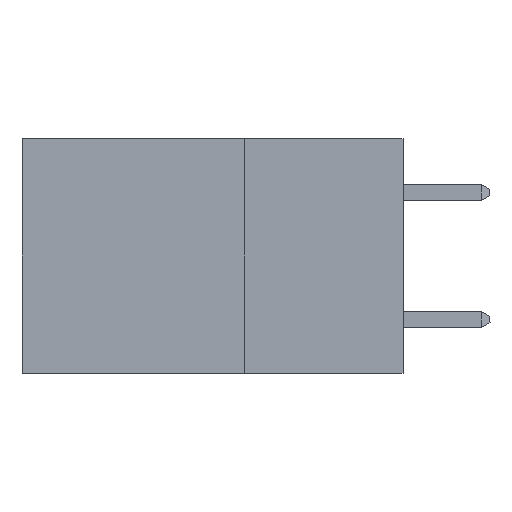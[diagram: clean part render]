
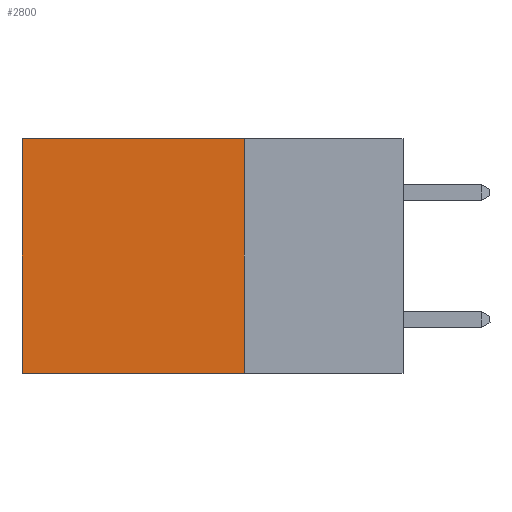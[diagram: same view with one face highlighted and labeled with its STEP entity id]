
A CAD part, left-side view. The second image highlights one B-rep face of the part: STEP entity #2800.
In plain terms, the highlighted planar face has unit normal (-1, 0, 0).
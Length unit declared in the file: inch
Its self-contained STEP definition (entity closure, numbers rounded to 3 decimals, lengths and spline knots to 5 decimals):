
#167 = AXIS2_PLACEMENT_3D ( 'NONE', #10324, #6565, #6544 ) ;
#244 = EDGE_CURVE ( 'NONE', #8905, #12550, #1825, .T. ) ;
#961 = LINE ( 'NONE', #6795, #11125 ) ;
#1372 = DIRECTION ( 'NONE',  ( 0., 1., 0. ) ) ;
#1406 = CARTESIAN_POINT ( 'NONE',  ( 0.2875, 0.25, -0.37 ) ) ;
#1825 = LINE ( 'NONE', #7615, #15183 ) ;
#2068 = ORIENTED_EDGE ( 'NONE', *, *, #244, .F. ) ;
#2527 = EDGE_CURVE ( 'NONE', #4469, #8905, #10467, .T. ) ;
#2800 = ADVANCED_FACE ( 'NONE', ( #6689 ), #5011, .F. ) ;
#3368 = VECTOR ( 'NONE', #6262, 39.37008 ) ;
#3665 = EDGE_LOOP ( 'NONE', ( #4724, #2068, #9142, #15760 ) ) ;
#4469 = VERTEX_POINT ( 'NONE', #9447 ) ;
#4653 = VECTOR ( 'NONE', #1372, 39.37008 ) ;
#4724 = ORIENTED_EDGE ( 'NONE', *, *, #15504, .T. ) ;
#5011 = PLANE ( 'NONE',  #167 ) ;
#5338 = CARTESIAN_POINT ( 'NONE',  ( 0.2875, 0.25, 0. ) ) ;
#5473 = DIRECTION ( 'NONE',  ( 0., 0., -1. ) ) ;
#6262 = DIRECTION ( 'NONE',  ( 0., 0., -1. ) ) ;
#6276 = DIRECTION ( 'NONE',  ( 0., 1., 0. ) ) ;
#6444 = CARTESIAN_POINT ( 'NONE',  ( 0.2875, 0.25, 0. ) ) ;
#6544 = DIRECTION ( 'NONE',  ( 0., 0., -1. ) ) ;
#6565 = DIRECTION ( 'NONE',  ( 1., 0., 0. ) ) ;
#6689 = FACE_OUTER_BOUND ( 'NONE', #3665, .T. ) ;
#6795 = CARTESIAN_POINT ( 'NONE',  ( 0.2875, 0.6, 0. ) ) ;
#7017 = VERTEX_POINT ( 'NONE', #8759 ) ;
#7615 = CARTESIAN_POINT ( 'NONE',  ( 0.2875, 0.25, -0.37 ) ) ;
#8759 = CARTESIAN_POINT ( 'NONE',  ( 0.2875, 0.6, 0. ) ) ;
#8905 = VERTEX_POINT ( 'NONE', #1406 ) ;
#9142 = ORIENTED_EDGE ( 'NONE', *, *, #2527, .F. ) ;
#9447 = CARTESIAN_POINT ( 'NONE',  ( 0.2875, 0.25, 0. ) ) ;
#10238 = EDGE_CURVE ( 'NONE', #4469, #7017, #14965, .T. ) ;
#10324 = CARTESIAN_POINT ( 'NONE',  ( 0.2875, 0.25, 0. ) ) ;
#10467 = LINE ( 'NONE', #6444, #3368 ) ;
#11125 = VECTOR ( 'NONE', #5473, 39.37008 ) ;
#12550 = VERTEX_POINT ( 'NONE', #16232 ) ;
#14965 = LINE ( 'NONE', #5338, #4653 ) ;
#15183 = VECTOR ( 'NONE', #6276, 39.37008 ) ;
#15504 = EDGE_CURVE ( 'NONE', #7017, #12550, #961, .T. ) ;
#15760 = ORIENTED_EDGE ( 'NONE', *, *, #10238, .T. ) ;
#16232 = CARTESIAN_POINT ( 'NONE',  ( 0.2875, 0.6, -0.37 ) ) ;
